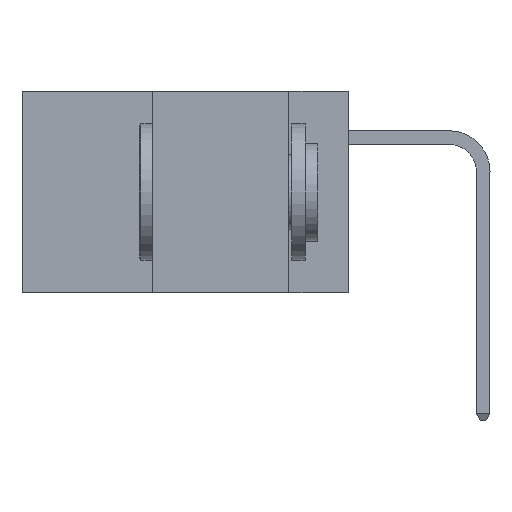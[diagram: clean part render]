
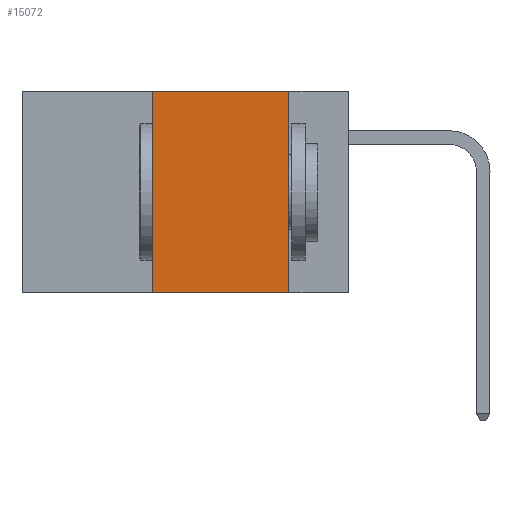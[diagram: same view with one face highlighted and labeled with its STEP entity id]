
A CAD part, left-side view. The second image highlights one B-rep face of the part: STEP entity #15072.
In plain terms, the highlighted planar face has unit normal (-1, 0, 0).
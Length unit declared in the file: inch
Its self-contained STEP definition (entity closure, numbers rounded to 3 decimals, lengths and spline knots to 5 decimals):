
#418 = DIRECTION ( 'NONE',  ( 0., 0., 1. ) ) ;
#619 = CARTESIAN_POINT ( 'NONE',  ( 0., 0.11, 0. ) ) ;
#864 = DIRECTION ( 'NONE',  ( 0., -1., 0. ) ) ;
#1143 = VERTEX_POINT ( 'NONE', #619 ) ;
#1177 = CARTESIAN_POINT ( 'NONE',  ( 0., 0.36, 0. ) ) ;
#2140 = EDGE_LOOP ( 'NONE', ( #14830, #17714, #23081, #15996 ) ) ;
#2515 = VECTOR ( 'NONE', #418, 39.37008 ) ;
#3345 = PLANE ( 'NONE',  #17938 ) ;
#3965 = DIRECTION ( 'NONE',  ( 0., -1., 0. ) ) ;
#5168 = CARTESIAN_POINT ( 'NONE',  ( 0., 0.11, 0. ) ) ;
#5200 = DIRECTION ( 'NONE',  ( 0., 0., -1. ) ) ;
#5769 = FACE_OUTER_BOUND ( 'NONE', #2140, .T. ) ;
#5815 = EDGE_CURVE ( 'NONE', #12582, #1143, #22138, .T. ) ;
#6270 = LINE ( 'NONE', #11570, #2515 ) ;
#7129 = DIRECTION ( 'NONE',  ( 0., 0., -1. ) ) ;
#7533 = VERTEX_POINT ( 'NONE', #19733 ) ;
#10118 = CARTESIAN_POINT ( 'NONE',  ( 0., 0.36, -0.37 ) ) ;
#11570 = CARTESIAN_POINT ( 'NONE',  ( 0., 0.36, 0. ) ) ;
#11916 = VECTOR ( 'NONE', #864, 39.37008 ) ;
#12582 = VERTEX_POINT ( 'NONE', #1177 ) ;
#14830 = ORIENTED_EDGE ( 'NONE', *, *, #16274, .F. ) ;
#15011 = CARTESIAN_POINT ( 'NONE',  ( 0., 0.6, -0.37 ) ) ;
#15072 = ADVANCED_FACE ( 'NONE', ( #5769 ), #3345, .F. ) ;
#15575 = CARTESIAN_POINT ( 'NONE',  ( 0., 0.6, 0. ) ) ;
#15694 = LINE ( 'NONE', #15011, #20521 ) ;
#15811 = LINE ( 'NONE', #5168, #18142 ) ;
#15996 = ORIENTED_EDGE ( 'NONE', *, *, #22758, .T. ) ;
#16166 = CARTESIAN_POINT ( 'NONE',  ( 0., 0.6, 0. ) ) ;
#16260 = DIRECTION ( 'NONE',  ( 1., 0., 0. ) ) ;
#16274 = EDGE_CURVE ( 'NONE', #1143, #7533, #15811, .T. ) ;
#16535 = VERTEX_POINT ( 'NONE', #10118 ) ;
#17008 = EDGE_CURVE ( 'NONE', #16535, #12582, #6270, .T. ) ;
#17714 = ORIENTED_EDGE ( 'NONE', *, *, #5815, .F. ) ;
#17938 = AXIS2_PLACEMENT_3D ( 'NONE', #16166, #16260, #5200 ) ;
#18142 = VECTOR ( 'NONE', #7129, 39.37008 ) ;
#19733 = CARTESIAN_POINT ( 'NONE',  ( 0., 0.11, -0.37 ) ) ;
#20521 = VECTOR ( 'NONE', #3965, 39.37008 ) ;
#22138 = LINE ( 'NONE', #15575, #11916 ) ;
#22758 = EDGE_CURVE ( 'NONE', #16535, #7533, #15694, .T. ) ;
#23081 = ORIENTED_EDGE ( 'NONE', *, *, #17008, .F. ) ;
